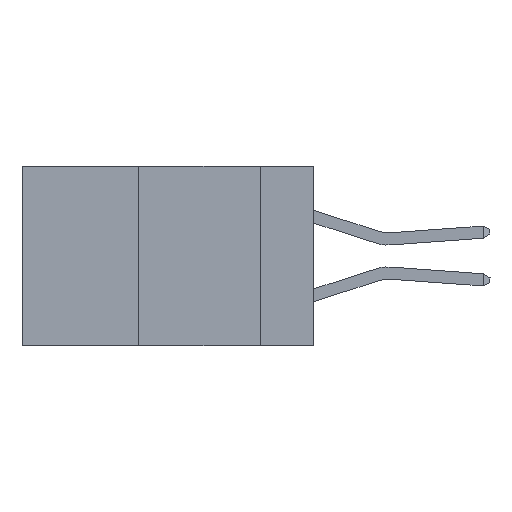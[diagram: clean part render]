
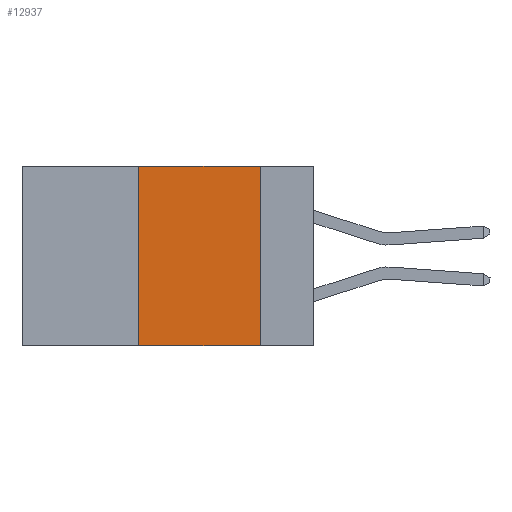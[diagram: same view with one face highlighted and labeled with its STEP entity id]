
A CAD part, left-side view. The second image highlights one B-rep face of the part: STEP entity #12937.
In plain terms, the highlighted planar face has unit normal (-1, 0, 0).
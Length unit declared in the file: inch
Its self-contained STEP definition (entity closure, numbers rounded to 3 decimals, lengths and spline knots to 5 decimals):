
#16 = DIRECTION ( 'NONE',  ( 0., -1., 0. ) ) ;
#745 = DIRECTION ( 'NONE',  ( 0., 0., -1. ) ) ;
#1045 = DIRECTION ( 'NONE',  ( 1., 0., 0. ) ) ;
#2850 = CARTESIAN_POINT ( 'NONE',  ( 0., 0.11, 0. ) ) ;
#2900 = ORIENTED_EDGE ( 'NONE', *, *, #4798, .F. ) ;
#3137 = DIRECTION ( 'NONE',  ( 0., 0., 1. ) ) ;
#3775 = FACE_OUTER_BOUND ( 'NONE', #7027, .T. ) ;
#4461 = VERTEX_POINT ( 'NONE', #11991 ) ;
#4798 = EDGE_CURVE ( 'NONE', #17417, #4461, #9835, .T. ) ;
#6119 = VERTEX_POINT ( 'NONE', #11604 ) ;
#6157 = VECTOR ( 'NONE', #745, 39.37008 ) ;
#6242 = EDGE_CURVE ( 'NONE', #6119, #17417, #8927, .T. ) ;
#6395 = LINE ( 'NONE', #19036, #17963 ) ;
#6480 = DIRECTION ( 'NONE',  ( 0., -1., 0. ) ) ;
#7027 = EDGE_LOOP ( 'NONE', ( #2900, #8987, #10027, #20162 ) ) ;
#7296 = LINE ( 'NONE', #23232, #16595 ) ;
#8927 = LINE ( 'NONE', #16213, #22512 ) ;
#8987 = ORIENTED_EDGE ( 'NONE', *, *, #6242, .F. ) ;
#9835 = LINE ( 'NONE', #13432, #6157 ) ;
#10027 = ORIENTED_EDGE ( 'NONE', *, *, #10897, .F. ) ;
#10425 = AXIS2_PLACEMENT_3D ( 'NONE', #17241, #1045, #17312 ) ;
#10897 = EDGE_CURVE ( 'NONE', #11615, #6119, #7296, .T. ) ;
#11604 = CARTESIAN_POINT ( 'NONE',  ( 0., 0.36, 0. ) ) ;
#11615 = VERTEX_POINT ( 'NONE', #14272 ) ;
#11991 = CARTESIAN_POINT ( 'NONE',  ( 0., 0.11, -0.37 ) ) ;
#12937 = ADVANCED_FACE ( 'NONE', ( #3775 ), #13651, .F. ) ;
#13432 = CARTESIAN_POINT ( 'NONE',  ( 0., 0.11, 0. ) ) ;
#13651 = PLANE ( 'NONE',  #10425 ) ;
#14272 = CARTESIAN_POINT ( 'NONE',  ( 0., 0.36, -0.37 ) ) ;
#16213 = CARTESIAN_POINT ( 'NONE',  ( 0., 0.6, 0. ) ) ;
#16595 = VECTOR ( 'NONE', #3137, 39.37008 ) ;
#17241 = CARTESIAN_POINT ( 'NONE',  ( 0., 0.6, 0. ) ) ;
#17312 = DIRECTION ( 'NONE',  ( 0., 0., -1. ) ) ;
#17417 = VERTEX_POINT ( 'NONE', #2850 ) ;
#17963 = VECTOR ( 'NONE', #6480, 39.37008 ) ;
#19036 = CARTESIAN_POINT ( 'NONE',  ( 0., 0.6, -0.37 ) ) ;
#20162 = ORIENTED_EDGE ( 'NONE', *, *, #23064, .T. ) ;
#22512 = VECTOR ( 'NONE', #16, 39.37008 ) ;
#23064 = EDGE_CURVE ( 'NONE', #11615, #4461, #6395, .T. ) ;
#23232 = CARTESIAN_POINT ( 'NONE',  ( 0., 0.36, 0. ) ) ;
